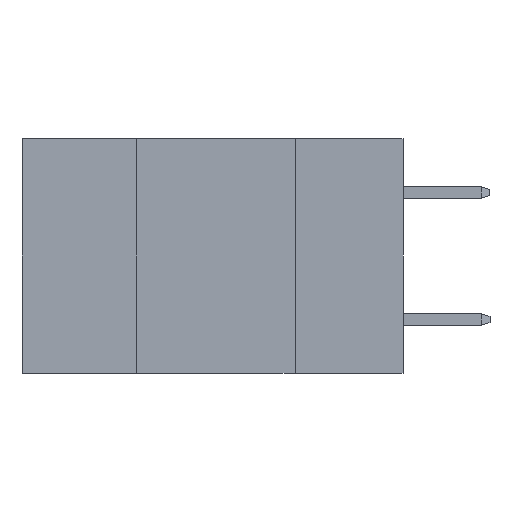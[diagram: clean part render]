
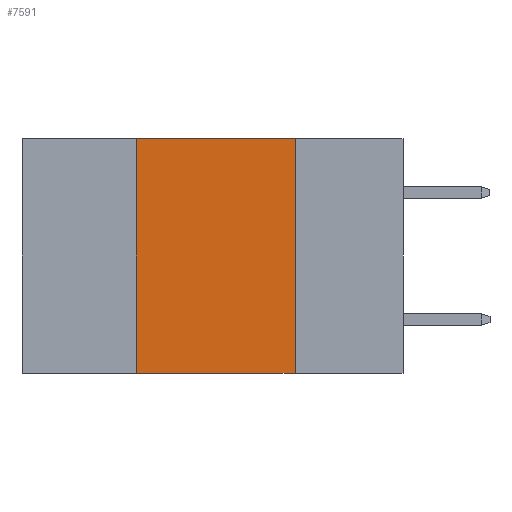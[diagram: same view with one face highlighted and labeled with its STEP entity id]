
A CAD part, left-side view. The second image highlights one B-rep face of the part: STEP entity #7591.
In plain terms, the highlighted planar face has unit normal (-1, 0, 0).
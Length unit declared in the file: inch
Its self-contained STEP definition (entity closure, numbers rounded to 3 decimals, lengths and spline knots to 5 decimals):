
#552 = EDGE_CURVE ( 'NONE', #914, #6838, #2186, .T. ) ;
#781 = CARTESIAN_POINT ( 'NONE',  ( 0., 0.6, 0. ) ) ;
#838 = EDGE_CURVE ( 'NONE', #3937, #5949, #9004, .T. ) ;
#914 = VERTEX_POINT ( 'NONE', #8676 ) ;
#939 = DIRECTION ( 'NONE',  ( 0., 0., 1. ) ) ;
#1482 = DIRECTION ( 'NONE',  ( 0., 0., -1. ) ) ;
#1676 = EDGE_CURVE ( 'NONE', #5949, #6838, #2663, .T. ) ;
#1774 = CARTESIAN_POINT ( 'NONE',  ( 0., 0.42, 0. ) ) ;
#2054 = VECTOR ( 'NONE', #2634, 39.37008 ) ;
#2186 = LINE ( 'NONE', #4996, #2620 ) ;
#2271 = ORIENTED_EDGE ( 'NONE', *, *, #4394, .F. ) ;
#2620 = VECTOR ( 'NONE', #5720, 39.37008 ) ;
#2634 = DIRECTION ( 'NONE',  ( 0., -1., 0. ) ) ;
#2663 = LINE ( 'NONE', #4781, #4144 ) ;
#3026 = LINE ( 'NONE', #1774, #7729 ) ;
#3556 = PLANE ( 'NONE',  #4527 ) ;
#3937 = VERTEX_POINT ( 'NONE', #5191 ) ;
#4144 = VECTOR ( 'NONE', #6105, 39.37008 ) ;
#4248 = FACE_OUTER_BOUND ( 'NONE', #8856, .T. ) ;
#4394 = EDGE_CURVE ( 'NONE', #914, #3937, #3026, .T. ) ;
#4527 = AXIS2_PLACEMENT_3D ( 'NONE', #781, #4987, #1482 ) ;
#4781 = CARTESIAN_POINT ( 'NONE',  ( 0., 0.17, 0. ) ) ;
#4987 = DIRECTION ( 'NONE',  ( 1., 0., 0. ) ) ;
#4996 = CARTESIAN_POINT ( 'NONE',  ( 0., 0.6, -0.37 ) ) ;
#5191 = CARTESIAN_POINT ( 'NONE',  ( 0., 0.42, 0. ) ) ;
#5582 = CARTESIAN_POINT ( 'NONE',  ( 0., 0.6, 0. ) ) ;
#5720 = DIRECTION ( 'NONE',  ( 0., -1., 0. ) ) ;
#5949 = VERTEX_POINT ( 'NONE', #7763 ) ;
#6105 = DIRECTION ( 'NONE',  ( 0., 0., -1. ) ) ;
#6838 = VERTEX_POINT ( 'NONE', #7740 ) ;
#7240 = ORIENTED_EDGE ( 'NONE', *, *, #552, .T. ) ;
#7591 = ADVANCED_FACE ( 'NONE', ( #4248 ), #3556, .F. ) ;
#7729 = VECTOR ( 'NONE', #939, 39.37008 ) ;
#7740 = CARTESIAN_POINT ( 'NONE',  ( 0., 0.17, -0.37 ) ) ;
#7763 = CARTESIAN_POINT ( 'NONE',  ( 0., 0.17, 0. ) ) ;
#8676 = CARTESIAN_POINT ( 'NONE',  ( 0., 0.42, -0.37 ) ) ;
#8750 = ORIENTED_EDGE ( 'NONE', *, *, #838, .F. ) ;
#8759 = ORIENTED_EDGE ( 'NONE', *, *, #1676, .F. ) ;
#8856 = EDGE_LOOP ( 'NONE', ( #8759, #8750, #2271, #7240 ) ) ;
#9004 = LINE ( 'NONE', #5582, #2054 ) ;
